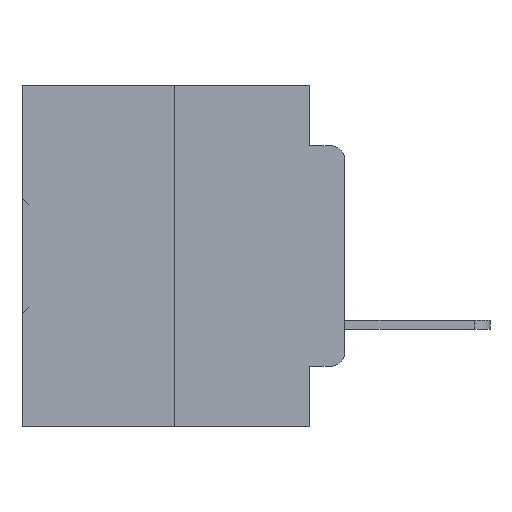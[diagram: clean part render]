
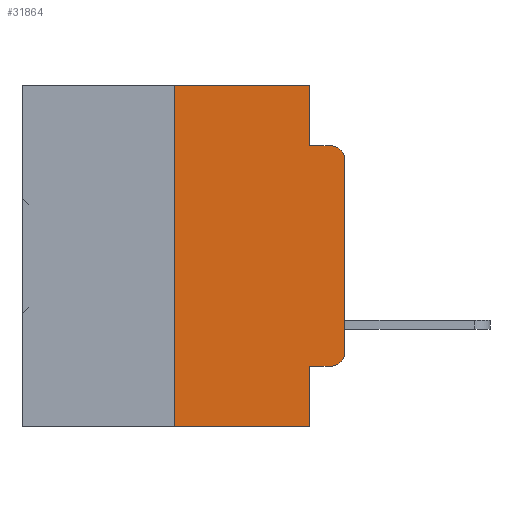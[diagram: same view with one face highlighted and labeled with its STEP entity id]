
A CAD part, left-side view. The second image highlights one B-rep face of the part: STEP entity #31864.
In plain terms, the highlighted planar face has unit normal (-1, 0, 0).
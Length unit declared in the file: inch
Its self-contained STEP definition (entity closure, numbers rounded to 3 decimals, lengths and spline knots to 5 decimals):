
#2 = CARTESIAN_POINT ( 'NONE',  ( 0., 0.02, -0.1085 ) ) ;
#265 = ORIENTED_EDGE ( 'NONE', *, *, #32533, .F. ) ;
#280 = CARTESIAN_POINT ( 'NONE',  ( 0., 0.473, 0. ) ) ;
#595 = DIRECTION ( 'NONE',  ( 0., 0., -1. ) ) ;
#1058 = CARTESIAN_POINT ( 'NONE',  ( 0., 0.02, -0.3915 ) ) ;
#1694 = EDGE_CURVE ( 'NONE', #29775, #4892, #19160, .T. ) ;
#1736 = EDGE_CURVE ( 'NONE', #13135, #11646, #11383, .T. ) ;
#1753 = CARTESIAN_POINT ( 'NONE',  ( 0., 0.02, -0.4115 ) ) ;
#1897 = VECTOR ( 'NONE', #18772, 39.37008 ) ;
#2487 = VECTOR ( 'NONE', #20410, 39.37008 ) ;
#2637 = ORIENTED_EDGE ( 'NONE', *, *, #14435, .F. ) ;
#2688 = CARTESIAN_POINT ( 'NONE',  ( 0., 0.473, -0.5 ) ) ;
#2806 = VECTOR ( 'NONE', #35396, 39.37008 ) ;
#2843 = LINE ( 'NONE', #31149, #32989 ) ;
#3064 = DIRECTION ( 'NONE',  ( 0., 0., -1. ) ) ;
#3318 = DIRECTION ( 'NONE',  ( 1., 0., 0. ) ) ;
#3452 = CARTESIAN_POINT ( 'NONE',  ( 0., 0.02, -0.0885 ) ) ;
#4049 = CARTESIAN_POINT ( 'NONE',  ( 0., 0.051, -0.4115 ) ) ;
#4051 = CARTESIAN_POINT ( 'NONE',  ( 0., 0.25, 0. ) ) ;
#4115 = DIRECTION ( 'NONE',  ( 0., 0., -1. ) ) ;
#4174 = CARTESIAN_POINT ( 'NONE',  ( 0., 0.051, -0.4115 ) ) ;
#4500 = EDGE_CURVE ( 'NONE', #13135, #7464, #23399, .T. ) ;
#4892 = VERTEX_POINT ( 'NONE', #33630 ) ;
#5198 = FACE_OUTER_BOUND ( 'NONE', #18356, .T. ) ;
#5498 = ORIENTED_EDGE ( 'NONE', *, *, #16379, .F. ) ;
#6263 = PLANE ( 'NONE',  #14668 ) ;
#6592 = AXIS2_PLACEMENT_3D ( 'NONE', #1058, #21777, #4115 ) ;
#7464 = VERTEX_POINT ( 'NONE', #4051 ) ;
#11383 = LINE ( 'NONE', #2688, #2487 ) ;
#11393 = LINE ( 'NONE', #18391, #25950 ) ;
#11646 = VERTEX_POINT ( 'NONE', #16133 ) ;
#11926 = CARTESIAN_POINT ( 'NONE',  ( 0., 0.051, 0. ) ) ;
#13135 = VERTEX_POINT ( 'NONE', #31696 ) ;
#13497 = LINE ( 'NONE', #11926, #34666 ) ;
#13787 = VERTEX_POINT ( 'NONE', #23284 ) ;
#13826 = ORIENTED_EDGE ( 'NONE', *, *, #20298, .F. ) ;
#14418 = DIRECTION ( 'NONE',  ( 0., 0., 1. ) ) ;
#14435 = EDGE_CURVE ( 'NONE', #27311, #13787, #11393, .T. ) ;
#14668 = AXIS2_PLACEMENT_3D ( 'NONE', #35249, #3318, #23889 ) ;
#15154 = EDGE_CURVE ( 'NONE', #26886, #29775, #17754, .T. ) ;
#15200 = ORIENTED_EDGE ( 'NONE', *, *, #1736, .T. ) ;
#15632 = CARTESIAN_POINT ( 'NONE',  ( 0., 0.051, 0. ) ) ;
#16133 = CARTESIAN_POINT ( 'NONE',  ( 0., 0.051, -0.5 ) ) ;
#16379 = EDGE_CURVE ( 'NONE', #7464, #27311, #34726, .T. ) ;
#16578 = VECTOR ( 'NONE', #34633, 39.37008 ) ;
#17510 = ORIENTED_EDGE ( 'NONE', *, *, #15154, .T. ) ;
#17754 = CIRCLE ( 'NONE', #6592, 0.02 ) ;
#17934 = DIRECTION ( 'NONE',  ( 0., 0., -1. ) ) ;
#18201 = VERTEX_POINT ( 'NONE', #3452 ) ;
#18315 = ORIENTED_EDGE ( 'NONE', *, *, #1694, .T. ) ;
#18356 = EDGE_LOOP ( 'NONE', ( #18315, #35397, #13826, #2637, #5498, #28772, #15200, #265, #30130, #17510 ) ) ;
#18391 = CARTESIAN_POINT ( 'NONE',  ( 0., 0.051, 0. ) ) ;
#18772 = DIRECTION ( 'NONE',  ( 0., -1., 0. ) ) ;
#19160 = LINE ( 'NONE', #31676, #27738 ) ;
#20298 = EDGE_CURVE ( 'NONE', #13787, #18201, #2843, .T. ) ;
#20410 = DIRECTION ( 'NONE',  ( 0., -1., 0. ) ) ;
#20437 = LINE ( 'NONE', #4049, #1897 ) ;
#20754 = DIRECTION ( 'NONE',  ( -1., 0., 0. ) ) ;
#20850 = CIRCLE ( 'NONE', #36546, 0.02 ) ;
#21777 = DIRECTION ( 'NONE',  ( -1., 0., 0. ) ) ;
#23284 = CARTESIAN_POINT ( 'NONE',  ( 0., 0.051, -0.0885 ) ) ;
#23399 = LINE ( 'NONE', #37446, #16578 ) ;
#23889 = DIRECTION ( 'NONE',  ( 0., 0., -1. ) ) ;
#24861 = EDGE_CURVE ( 'NONE', #24902, #26886, #20437, .T. ) ;
#24902 = VERTEX_POINT ( 'NONE', #4174 ) ;
#25950 = VECTOR ( 'NONE', #595, 39.37008 ) ;
#26886 = VERTEX_POINT ( 'NONE', #1753 ) ;
#27311 = VERTEX_POINT ( 'NONE', #15632 ) ;
#27738 = VECTOR ( 'NONE', #14418, 39.37008 ) ;
#28772 = ORIENTED_EDGE ( 'NONE', *, *, #4500, .F. ) ;
#29775 = VERTEX_POINT ( 'NONE', #33677 ) ;
#30130 = ORIENTED_EDGE ( 'NONE', *, *, #24861, .T. ) ;
#31149 = CARTESIAN_POINT ( 'NONE',  ( 0., 0.051, -0.0885 ) ) ;
#31676 = CARTESIAN_POINT ( 'NONE',  ( 0., 0., 0. ) ) ;
#31696 = CARTESIAN_POINT ( 'NONE',  ( 0., 0.25, -0.5 ) ) ;
#31819 = EDGE_CURVE ( 'NONE', #4892, #18201, #20850, .T. ) ;
#31864 = ADVANCED_FACE ( 'NONE', ( #5198 ), #6263, .F. ) ;
#32533 = EDGE_CURVE ( 'NONE', #24902, #11646, #13497, .T. ) ;
#32989 = VECTOR ( 'NONE', #36839, 39.37008 ) ;
#33630 = CARTESIAN_POINT ( 'NONE',  ( 0., 0., -0.1085 ) ) ;
#33677 = CARTESIAN_POINT ( 'NONE',  ( 0., 0., -0.3915 ) ) ;
#34633 = DIRECTION ( 'NONE',  ( 0., 0., 1. ) ) ;
#34666 = VECTOR ( 'NONE', #17934, 39.37008 ) ;
#34726 = LINE ( 'NONE', #280, #2806 ) ;
#35249 = CARTESIAN_POINT ( 'NONE',  ( 0., 0.473, 0. ) ) ;
#35396 = DIRECTION ( 'NONE',  ( 0., -1., 0. ) ) ;
#35397 = ORIENTED_EDGE ( 'NONE', *, *, #31819, .T. ) ;
#36546 = AXIS2_PLACEMENT_3D ( 'NONE', #2, #20754, #3064 ) ;
#36839 = DIRECTION ( 'NONE',  ( 0., -1., 0. ) ) ;
#37446 = CARTESIAN_POINT ( 'NONE',  ( 0., 0.25, 0. ) ) ;
